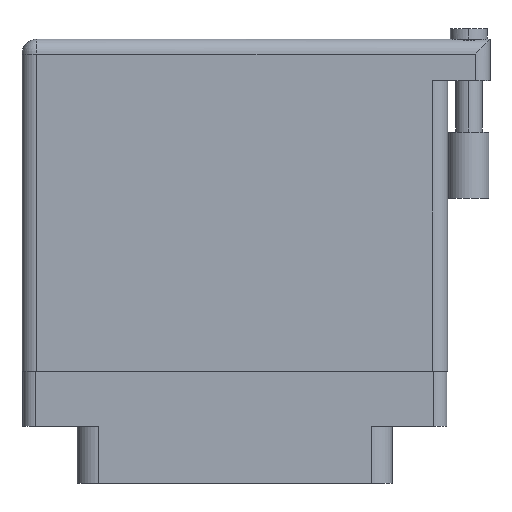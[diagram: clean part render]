
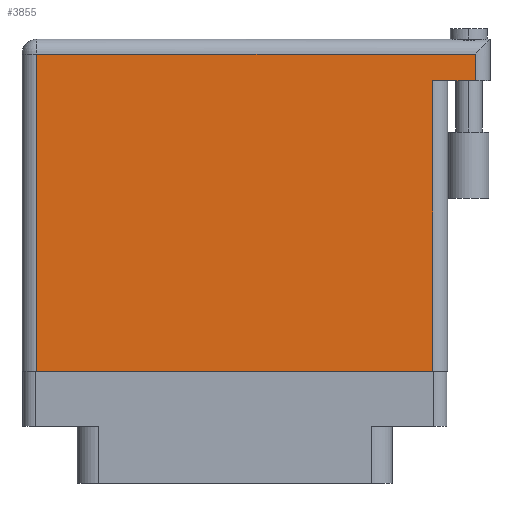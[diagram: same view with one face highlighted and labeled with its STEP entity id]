
A CAD part, front view. The second image highlights one B-rep face of the part: STEP entity #3855.
In plain terms, the highlighted face is planar.
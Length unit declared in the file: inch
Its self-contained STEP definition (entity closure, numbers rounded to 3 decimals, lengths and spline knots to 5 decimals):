
#681 = VECTOR ( 'NONE', #14847, 39.37008 ) ;
#890 = DIRECTION ( 'NONE',  ( 0., -1., 0. ) ) ;
#1549 = FACE_OUTER_BOUND ( 'NONE', #21491, .T. ) ;
#1730 = DIRECTION ( 'NONE',  ( 1., 0., 0. ) ) ;
#2799 = DIRECTION ( 'NONE',  ( -1., 0., 0. ) ) ;
#3101 = VERTEX_POINT ( 'NONE', #8050 ) ;
#3380 = CARTESIAN_POINT ( 'NONE',  ( 0., 1.496, 0. ) ) ;
#3855 = ADVANCED_FACE ( 'NONE', ( #1549 ), #21822, .F. ) ;
#4731 = LINE ( 'NONE', #5548, #681 ) ;
#4734 = VECTOR ( 'NONE', #890, 39.37008 ) ;
#5492 = EDGE_CURVE ( 'NONE', #18498, #6932, #27096, .T. ) ;
#5548 = CARTESIAN_POINT ( 'NONE',  ( 2.138, 1.566, 0. ) ) ;
#6932 = VERTEX_POINT ( 'NONE', #28692 ) ;
#6964 = VECTOR ( 'NONE', #1730, 39.37008 ) ;
#8050 = CARTESIAN_POINT ( 'NONE',  ( 1.938, 1.369, 0. ) ) ;
#8308 = CARTESIAN_POINT ( 'NONE',  ( 0.07, 1.496, 0. ) ) ;
#8585 = VECTOR ( 'NONE', #22960, 39.37008 ) ;
#8698 = EDGE_CURVE ( 'NONE', #12944, #18498, #11488, .T. ) ;
#9476 = VERTEX_POINT ( 'NONE', #22245 ) ;
#10869 = ORIENTED_EDGE ( 'NONE', *, *, #23864, .T. ) ;
#10905 = ORIENTED_EDGE ( 'NONE', *, *, #8698, .T. ) ;
#11488 = LINE ( 'NONE', #12308, #4734 ) ;
#11537 = AXIS2_PLACEMENT_3D ( 'NONE', #19879, #24658, #2799 ) ;
#12308 = CARTESIAN_POINT ( 'NONE',  ( 0.07, 0., 0. ) ) ;
#12551 = EDGE_CURVE ( 'NONE', #9476, #3101, #18741, .T. ) ;
#12944 = VERTEX_POINT ( 'NONE', #8308 ) ;
#13122 = ORIENTED_EDGE ( 'NONE', *, *, #12551, .F. ) ;
#13147 = LINE ( 'NONE', #16242, #24282 ) ;
#13902 = DIRECTION ( 'NONE',  ( -1., 0., 0. ) ) ;
#14106 = ORIENTED_EDGE ( 'NONE', *, *, #5492, .T. ) ;
#14847 = DIRECTION ( 'NONE',  ( 0., 1., 0. ) ) ;
#15837 = DIRECTION ( 'NONE',  ( 0., 1., 0. ) ) ;
#16046 = EDGE_CURVE ( 'NONE', #6932, #3101, #13147, .T. ) ;
#16242 = CARTESIAN_POINT ( 'NONE',  ( 1.938, 1.369, 0. ) ) ;
#16831 = LINE ( 'NONE', #3380, #8585 ) ;
#17625 = VERTEX_POINT ( 'NONE', #20894 ) ;
#18436 = ORIENTED_EDGE ( 'NONE', *, *, #16046, .T. ) ;
#18498 = VERTEX_POINT ( 'NONE', #27073 ) ;
#18741 = LINE ( 'NONE', #30815, #22442 ) ;
#19879 = CARTESIAN_POINT ( 'NONE',  ( 0., 1.566, 0. ) ) ;
#20894 = CARTESIAN_POINT ( 'NONE',  ( 2.138, 1.496, 0. ) ) ;
#21491 = EDGE_LOOP ( 'NONE', ( #14106, #18436, #13122, #10869, #22740, #10905 ) ) ;
#21822 = PLANE ( 'NONE',  #11537 ) ;
#22245 = CARTESIAN_POINT ( 'NONE',  ( 2.138, 1.369, 0. ) ) ;
#22442 = VECTOR ( 'NONE', #13902, 39.37008 ) ;
#22740 = ORIENTED_EDGE ( 'NONE', *, *, #28756, .T. ) ;
#22960 = DIRECTION ( 'NONE',  ( -1., 0., 0. ) ) ;
#23864 = EDGE_CURVE ( 'NONE', #9476, #17625, #4731, .T. ) ;
#24282 = VECTOR ( 'NONE', #15837, 39.37008 ) ;
#24658 = DIRECTION ( 'NONE',  ( 0., 0., -1. ) ) ;
#27073 = CARTESIAN_POINT ( 'NONE',  ( 0.07, 0., 0. ) ) ;
#27096 = LINE ( 'NONE', #27932, #6964 ) ;
#27932 = CARTESIAN_POINT ( 'NONE',  ( 0., 0., 0. ) ) ;
#28692 = CARTESIAN_POINT ( 'NONE',  ( 1.938, 0., 0. ) ) ;
#28756 = EDGE_CURVE ( 'NONE', #17625, #12944, #16831, .T. ) ;
#30815 = CARTESIAN_POINT ( 'NONE',  ( 2.208, 1.369, 0. ) ) ;
